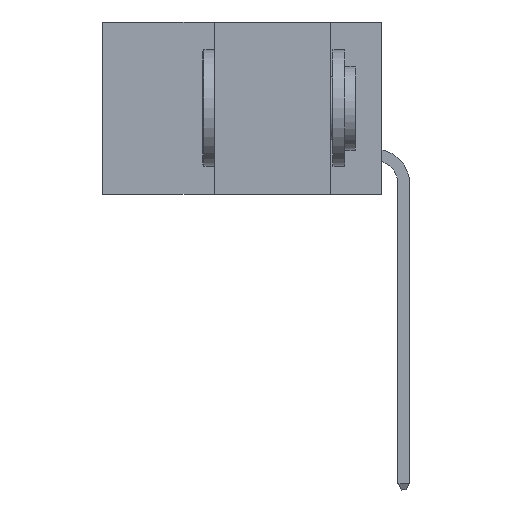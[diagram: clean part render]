
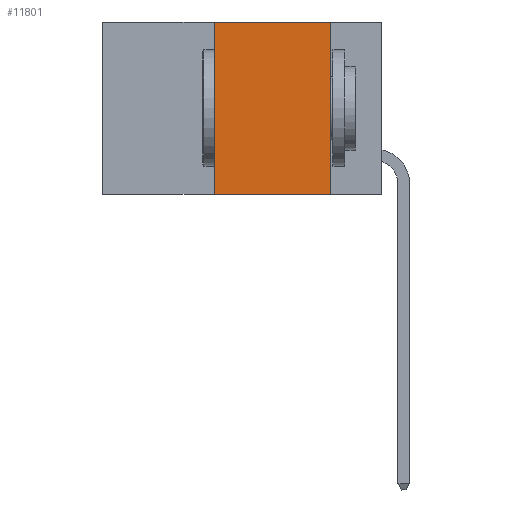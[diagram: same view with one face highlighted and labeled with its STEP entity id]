
A CAD part, left-side view. The second image highlights one B-rep face of the part: STEP entity #11801.
In plain terms, the highlighted planar face has unit normal (-1, 0, 0).
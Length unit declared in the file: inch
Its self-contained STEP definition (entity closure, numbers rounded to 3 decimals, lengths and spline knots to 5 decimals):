
#809 = CARTESIAN_POINT ( 'NONE',  ( 0., 0.6, -0.37 ) ) ;
#1384 = VECTOR ( 'NONE', #13293, 39.37008 ) ;
#1506 = PLANE ( 'NONE',  #5369 ) ;
#1825 = VECTOR ( 'NONE', #7439, 39.37008 ) ;
#1880 = CARTESIAN_POINT ( 'NONE',  ( 0., 0.36, -0.37 ) ) ;
#3077 = CARTESIAN_POINT ( 'NONE',  ( 0., 0.36, 0. ) ) ;
#3111 = DIRECTION ( 'NONE',  ( 1., 0., 0. ) ) ;
#3595 = CARTESIAN_POINT ( 'NONE',  ( 0., 0.36, 0. ) ) ;
#4232 = CARTESIAN_POINT ( 'NONE',  ( 0., 0.6, 0. ) ) ;
#5369 = AXIS2_PLACEMENT_3D ( 'NONE', #12466, #3111, #13879 ) ;
#5588 = CARTESIAN_POINT ( 'NONE',  ( 0., 0.11, 0. ) ) ;
#5786 = VERTEX_POINT ( 'NONE', #5588 ) ;
#6096 = LINE ( 'NONE', #4232, #1825 ) ;
#6098 = ORIENTED_EDGE ( 'NONE', *, *, #16212, .F. ) ;
#6363 = ORIENTED_EDGE ( 'NONE', *, *, #17699, .F. ) ;
#7326 = ORIENTED_EDGE ( 'NONE', *, *, #14726, .F. ) ;
#7439 = DIRECTION ( 'NONE',  ( 0., -1., 0. ) ) ;
#8218 = FACE_OUTER_BOUND ( 'NONE', #8363, .T. ) ;
#8363 = EDGE_LOOP ( 'NONE', ( #7326, #6098, #6363, #9096 ) ) ;
#8789 = VERTEX_POINT ( 'NONE', #3595 ) ;
#9096 = ORIENTED_EDGE ( 'NONE', *, *, #14942, .T. ) ;
#10135 = VECTOR ( 'NONE', #16654, 39.37008 ) ;
#10827 = LINE ( 'NONE', #809, #1384 ) ;
#11281 = CARTESIAN_POINT ( 'NONE',  ( 0., 0.11, -0.37 ) ) ;
#11801 = ADVANCED_FACE ( 'NONE', ( #8218 ), #1506, .F. ) ;
#12466 = CARTESIAN_POINT ( 'NONE',  ( 0., 0.6, 0. ) ) ;
#12773 = LINE ( 'NONE', #3077, #15576 ) ;
#13293 = DIRECTION ( 'NONE',  ( 0., -1., 0. ) ) ;
#13783 = DIRECTION ( 'NONE',  ( 0., 0., 1. ) ) ;
#13879 = DIRECTION ( 'NONE',  ( 0., 0., -1. ) ) ;
#13976 = LINE ( 'NONE', #19454, #10135 ) ;
#14726 = EDGE_CURVE ( 'NONE', #5786, #15898, #13976, .T. ) ;
#14942 = EDGE_CURVE ( 'NONE', #17233, #15898, #10827, .T. ) ;
#15576 = VECTOR ( 'NONE', #13783, 39.37008 ) ;
#15898 = VERTEX_POINT ( 'NONE', #11281 ) ;
#16212 = EDGE_CURVE ( 'NONE', #8789, #5786, #6096, .T. ) ;
#16654 = DIRECTION ( 'NONE',  ( 0., 0., -1. ) ) ;
#17233 = VERTEX_POINT ( 'NONE', #1880 ) ;
#17699 = EDGE_CURVE ( 'NONE', #17233, #8789, #12773, .T. ) ;
#19454 = CARTESIAN_POINT ( 'NONE',  ( 0., 0.11, 0. ) ) ;
